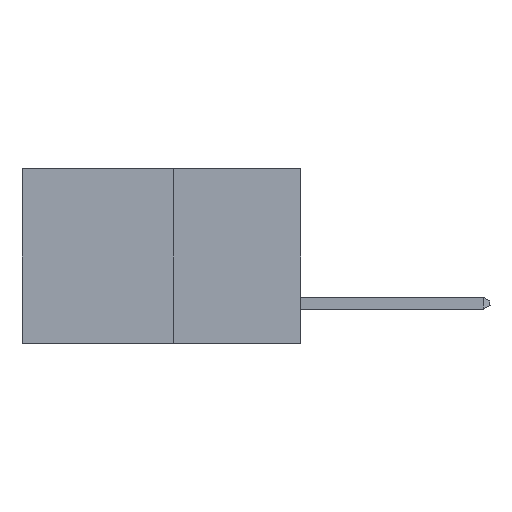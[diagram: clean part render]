
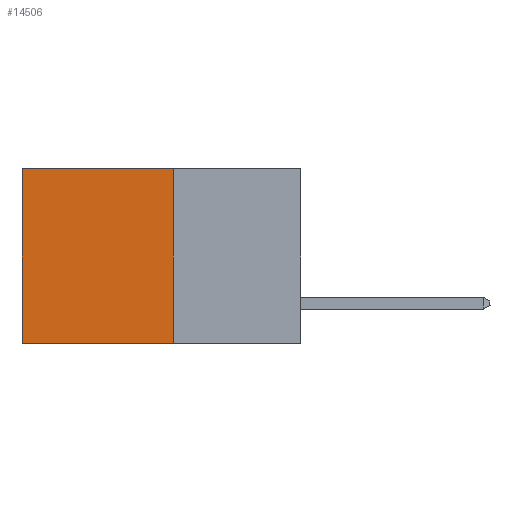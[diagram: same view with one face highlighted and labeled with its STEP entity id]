
A CAD part, left-side view. The second image highlights one B-rep face of the part: STEP entity #14506.
In plain terms, the highlighted planar face has unit normal (-1, 0, 0).
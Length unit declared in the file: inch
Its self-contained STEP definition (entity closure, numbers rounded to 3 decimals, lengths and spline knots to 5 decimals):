
#16 = CARTESIAN_POINT ( 'NONE',  ( 0.277, 0.27, -0.37 ) ) ;
#49 = VECTOR ( 'NONE', #19444, 39.37008 ) ;
#510 = CARTESIAN_POINT ( 'NONE',  ( 0.277, 0.27, -0.37 ) ) ;
#565 = DIRECTION ( 'NONE',  ( 0., 0., -1. ) ) ;
#1057 = CARTESIAN_POINT ( 'NONE',  ( 0.277, 0.59, -0.37 ) ) ;
#1814 = VECTOR ( 'NONE', #565, 39.37008 ) ;
#2205 = EDGE_CURVE ( 'NONE', #3220, #14812, #11821, .T. ) ;
#2303 = EDGE_CURVE ( 'NONE', #3220, #7941, #4862, .T. ) ;
#3220 = VERTEX_POINT ( 'NONE', #19993 ) ;
#3549 = ORIENTED_EDGE ( 'NONE', *, *, #2303, .T. ) ;
#4093 = ORIENTED_EDGE ( 'NONE', *, *, #11767, .F. ) ;
#4591 = ORIENTED_EDGE ( 'NONE', *, *, #2205, .F. ) ;
#4783 = LINE ( 'NONE', #16, #49 ) ;
#4862 = LINE ( 'NONE', #9131, #17824 ) ;
#5148 = CARTESIAN_POINT ( 'NONE',  ( 0.277, 0.27, -0.37 ) ) ;
#7941 = VERTEX_POINT ( 'NONE', #17940 ) ;
#8561 = DIRECTION ( 'NONE',  ( 1., 0., 0. ) ) ;
#9131 = CARTESIAN_POINT ( 'NONE',  ( 0.277, 0.27, 0. ) ) ;
#9835 = DIRECTION ( 'NONE',  ( 0., 1., 0. ) ) ;
#10359 = VERTEX_POINT ( 'NONE', #10560 ) ;
#10560 = CARTESIAN_POINT ( 'NONE',  ( 0.277, 0.59, -0.37 ) ) ;
#11767 = EDGE_CURVE ( 'NONE', #14812, #10359, #4783, .T. ) ;
#11821 = LINE ( 'NONE', #5148, #1814 ) ;
#11905 = ORIENTED_EDGE ( 'NONE', *, *, #21107, .T. ) ;
#12290 = AXIS2_PLACEMENT_3D ( 'NONE', #22326, #8561, #20791 ) ;
#14131 = LINE ( 'NONE', #1057, #18217 ) ;
#14506 = ADVANCED_FACE ( 'NONE', ( #14897 ), #19089, .F. ) ;
#14812 = VERTEX_POINT ( 'NONE', #510 ) ;
#14897 = FACE_OUTER_BOUND ( 'NONE', #19090, .T. ) ;
#15213 = DIRECTION ( 'NONE',  ( 0., 0., -1. ) ) ;
#17824 = VECTOR ( 'NONE', #9835, 39.37008 ) ;
#17940 = CARTESIAN_POINT ( 'NONE',  ( 0.277, 0.59, 0. ) ) ;
#18217 = VECTOR ( 'NONE', #15213, 39.37008 ) ;
#19089 = PLANE ( 'NONE',  #12290 ) ;
#19090 = EDGE_LOOP ( 'NONE', ( #11905, #4093, #4591, #3549 ) ) ;
#19444 = DIRECTION ( 'NONE',  ( 0., 1., 0. ) ) ;
#19993 = CARTESIAN_POINT ( 'NONE',  ( 0.277, 0.27, 0. ) ) ;
#20791 = DIRECTION ( 'NONE',  ( 0., 0., -1. ) ) ;
#21107 = EDGE_CURVE ( 'NONE', #7941, #10359, #14131, .T. ) ;
#22326 = CARTESIAN_POINT ( 'NONE',  ( 0.277, 0.27, -0.37 ) ) ;
